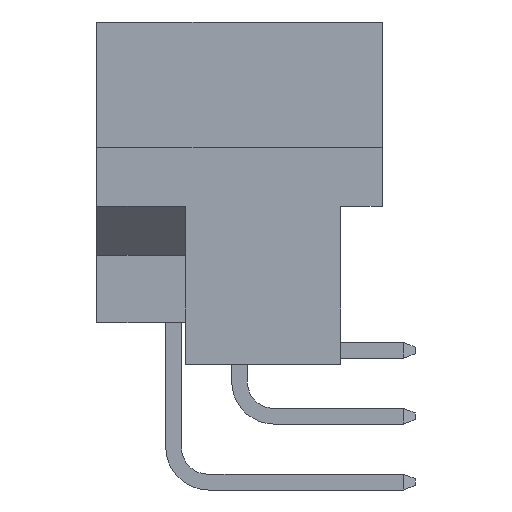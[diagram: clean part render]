
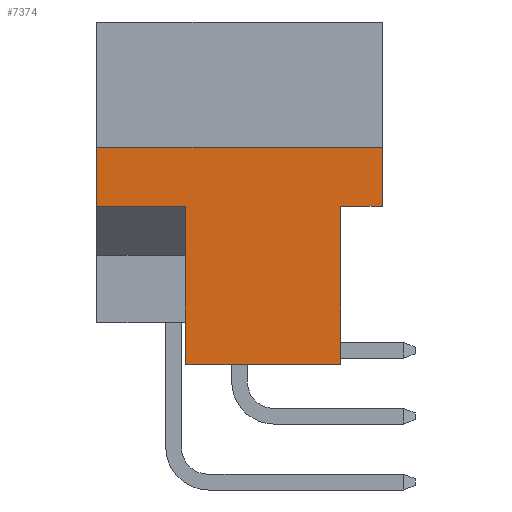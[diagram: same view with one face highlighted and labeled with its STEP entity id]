
A CAD part, left-side view. The second image highlights one B-rep face of the part: STEP entity #7374.
In plain terms, the highlighted planar face has unit normal (-1, 0, 0).
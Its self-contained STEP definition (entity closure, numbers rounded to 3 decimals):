
#226 = VECTOR ( 'NONE', #4537, 1000. ) ;
#500 = VERTEX_POINT ( 'NONE', #2143 ) ;
#546 = CARTESIAN_POINT ( 'NONE',  ( 0., 10.998, -13.2 ) ) ;
#852 = ORIENTED_EDGE ( 'NONE', *, *, #8110, .F. ) ;
#1022 = PLANE ( 'NONE',  #7591 ) ;
#1117 = CARTESIAN_POINT ( 'NONE',  ( 0., 7.597, -7.112 ) ) ;
#1143 = EDGE_CURVE ( 'NONE', #9324, #7468, #3123, .T. ) ;
#1316 = LINE ( 'NONE', #1117, #8181 ) ;
#1465 = CARTESIAN_POINT ( 'NONE',  ( 0., 1.6, 46.912 ) ) ;
#1496 = CARTESIAN_POINT ( 'NONE',  ( 0., 10.998, 0. ) ) ;
#1498 = CARTESIAN_POINT ( 'NONE',  ( 0., 1.6, -7.112 ) ) ;
#1769 = CARTESIAN_POINT ( 'NONE',  ( 0., 10.998, -7.112 ) ) ;
#1921 = FACE_OUTER_BOUND ( 'NONE', #2098, .T. ) ;
#1932 = CARTESIAN_POINT ( 'NONE',  ( 0., 0., 0. ) ) ;
#2004 = VERTEX_POINT ( 'NONE', #7792 ) ;
#2098 = EDGE_LOOP ( 'NONE', ( #2576, #6557, #7501, #9239, #852, #3600, #8320, #8708 ) ) ;
#2143 = CARTESIAN_POINT ( 'NONE',  ( 0., 7.597, -13.2 ) ) ;
#2260 = LINE ( 'NONE', #3011, #4552 ) ;
#2576 = ORIENTED_EDGE ( 'NONE', *, *, #1143, .F. ) ;
#2630 = CARTESIAN_POINT ( 'NONE',  ( 0., 10.998, 0. ) ) ;
#2834 = CARTESIAN_POINT ( 'NONE',  ( 0., 7.597, -13.2 ) ) ;
#3011 = CARTESIAN_POINT ( 'NONE',  ( 0., 10.998, -4.826 ) ) ;
#3123 = LINE ( 'NONE', #1465, #6176 ) ;
#3600 = ORIENTED_EDGE ( 'NONE', *, *, #6653, .F. ) ;
#3603 = VECTOR ( 'NONE', #4644, 1000. ) ;
#3685 = CARTESIAN_POINT ( 'NONE',  ( 0., 0., -7.112 ) ) ;
#3807 = EDGE_CURVE ( 'NONE', #500, #8354, #8834, .T. ) ;
#3843 = EDGE_CURVE ( 'NONE', #4404, #5889, #8885, .T. ) ;
#3968 = DIRECTION ( 'NONE',  ( 0., 0., -1. ) ) ;
#4141 = CARTESIAN_POINT ( 'NONE',  ( 0., 7.597, -7.112 ) ) ;
#4404 = VERTEX_POINT ( 'NONE', #5393 ) ;
#4511 = DIRECTION ( 'NONE',  ( 0., -1., 0. ) ) ;
#4537 = DIRECTION ( 'NONE',  ( 0., 1., 0. ) ) ;
#4552 = VECTOR ( 'NONE', #4511, 1000. ) ;
#4644 = DIRECTION ( 'NONE',  ( 0., 0., 1. ) ) ;
#4757 = EDGE_CURVE ( 'NONE', #500, #7468, #4998, .T. ) ;
#4937 = EDGE_CURVE ( 'NONE', #4404, #9324, #7639, .T. ) ;
#4998 = LINE ( 'NONE', #546, #9158 ) ;
#5084 = DIRECTION ( 'NONE',  ( 0., 0., 1. ) ) ;
#5320 = VECTOR ( 'NONE', #6539, 1000. ) ;
#5364 = DIRECTION ( 'NONE',  ( 0., 0., -1. ) ) ;
#5393 = CARTESIAN_POINT ( 'NONE',  ( 0., 0., -7.112 ) ) ;
#5889 = VERTEX_POINT ( 'NONE', #8863 ) ;
#6176 = VECTOR ( 'NONE', #5364, 1000. ) ;
#6483 = CARTESIAN_POINT ( 'NONE',  ( 0., 1.6, -13.2 ) ) ;
#6539 = DIRECTION ( 'NONE',  ( 0., 0., 1. ) ) ;
#6555 = VERTEX_POINT ( 'NONE', #1769 ) ;
#6557 = ORIENTED_EDGE ( 'NONE', *, *, #4937, .F. ) ;
#6653 = EDGE_CURVE ( 'NONE', #8354, #6555, #1316, .T. ) ;
#7374 = ADVANCED_FACE ( 'NONE', ( #1921 ), #1022, .F. ) ;
#7468 = VERTEX_POINT ( 'NONE', #6483 ) ;
#7501 = ORIENTED_EDGE ( 'NONE', *, *, #3843, .T. ) ;
#7591 = AXIS2_PLACEMENT_3D ( 'NONE', #2630, #7923, #3968 ) ;
#7639 = LINE ( 'NONE', #3685, #226 ) ;
#7658 = EDGE_CURVE ( 'NONE', #2004, #5889, #2260, .T. ) ;
#7792 = CARTESIAN_POINT ( 'NONE',  ( 0., 10.998, -4.826 ) ) ;
#7923 = DIRECTION ( 'NONE',  ( 1., 0., 0. ) ) ;
#8110 = EDGE_CURVE ( 'NONE', #6555, #2004, #9193, .T. ) ;
#8181 = VECTOR ( 'NONE', #9578, 1000. ) ;
#8320 = ORIENTED_EDGE ( 'NONE', *, *, #3807, .F. ) ;
#8354 = VERTEX_POINT ( 'NONE', #4141 ) ;
#8708 = ORIENTED_EDGE ( 'NONE', *, *, #4757, .T. ) ;
#8834 = LINE ( 'NONE', #2834, #9641 ) ;
#8863 = CARTESIAN_POINT ( 'NONE',  ( 0., 0., -4.826 ) ) ;
#8885 = LINE ( 'NONE', #1932, #5320 ) ;
#9158 = VECTOR ( 'NONE', #9738, 1000. ) ;
#9193 = LINE ( 'NONE', #1496, #3603 ) ;
#9239 = ORIENTED_EDGE ( 'NONE', *, *, #7658, .F. ) ;
#9324 = VERTEX_POINT ( 'NONE', #1498 ) ;
#9578 = DIRECTION ( 'NONE',  ( 0., 1., 0. ) ) ;
#9641 = VECTOR ( 'NONE', #5084, 1000. ) ;
#9738 = DIRECTION ( 'NONE',  ( 0., -1., 0. ) ) ;
